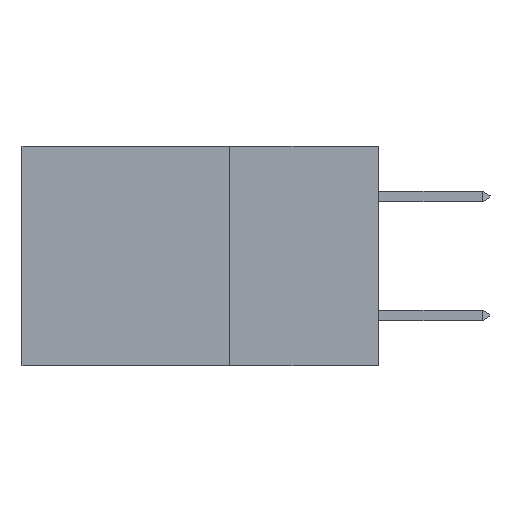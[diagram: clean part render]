
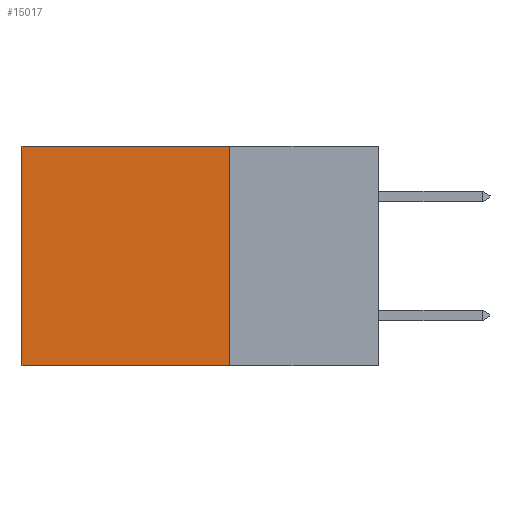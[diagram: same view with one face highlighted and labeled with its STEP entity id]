
A CAD part, left-side view. The second image highlights one B-rep face of the part: STEP entity #15017.
In plain terms, the highlighted planar face has unit normal (-1, 0, 0).
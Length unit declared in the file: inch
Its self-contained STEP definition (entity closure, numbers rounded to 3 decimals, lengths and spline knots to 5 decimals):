
#1255 = CARTESIAN_POINT ( 'NONE',  ( 0.2615, 0.6, -0.37 ) ) ;
#1549 = ORIENTED_EDGE ( 'NONE', *, *, #15933, .F. ) ;
#3287 = CARTESIAN_POINT ( 'NONE',  ( 0.2615, 0.6, 0. ) ) ;
#3736 = VERTEX_POINT ( 'NONE', #17501 ) ;
#4346 = VECTOR ( 'NONE', #14402, 39.37008 ) ;
#4404 = LINE ( 'NONE', #11683, #4346 ) ;
#4948 = EDGE_CURVE ( 'NONE', #3736, #9609, #12478, .T. ) ;
#5705 = EDGE_LOOP ( 'NONE', ( #17864, #1549, #15729, #14238 ) ) ;
#5894 = DIRECTION ( 'NONE',  ( 1., 0., 0. ) ) ;
#7299 = CARTESIAN_POINT ( 'NONE',  ( 0.2615, 0.25, -0.37 ) ) ;
#7676 = EDGE_CURVE ( 'NONE', #3736, #17178, #4404, .T. ) ;
#8292 = CARTESIAN_POINT ( 'NONE',  ( 0.2615, 0.25, 0. ) ) ;
#8500 = CARTESIAN_POINT ( 'NONE',  ( 0.2615, 0.25, -0.37 ) ) ;
#8706 = FACE_OUTER_BOUND ( 'NONE', #5705, .T. ) ;
#9117 = LINE ( 'NONE', #10249, #13138 ) ;
#9609 = VERTEX_POINT ( 'NONE', #3287 ) ;
#10249 = CARTESIAN_POINT ( 'NONE',  ( 0.2615, 0.25, -0.37 ) ) ;
#10652 = LINE ( 'NONE', #12328, #11546 ) ;
#10745 = DIRECTION ( 'NONE',  ( 0., 0., -1. ) ) ;
#11460 = EDGE_CURVE ( 'NONE', #9609, #15410, #10652, .T. ) ;
#11546 = VECTOR ( 'NONE', #10745, 39.37008 ) ;
#11683 = CARTESIAN_POINT ( 'NONE',  ( 0.2615, 0.25, -0.37 ) ) ;
#12328 = CARTESIAN_POINT ( 'NONE',  ( 0.2615, 0.6, -0.37 ) ) ;
#12478 = LINE ( 'NONE', #8292, #17111 ) ;
#12896 = DIRECTION ( 'NONE',  ( 0., 0., -1. ) ) ;
#13138 = VECTOR ( 'NONE', #14911, 39.37008 ) ;
#13408 = AXIS2_PLACEMENT_3D ( 'NONE', #7299, #5894, #12896 ) ;
#14238 = ORIENTED_EDGE ( 'NONE', *, *, #4948, .T. ) ;
#14402 = DIRECTION ( 'NONE',  ( 0., 0., -1. ) ) ;
#14911 = DIRECTION ( 'NONE',  ( 0., 1., 0. ) ) ;
#15017 = ADVANCED_FACE ( 'NONE', ( #8706 ), #17397, .F. ) ;
#15410 = VERTEX_POINT ( 'NONE', #1255 ) ;
#15729 = ORIENTED_EDGE ( 'NONE', *, *, #7676, .F. ) ;
#15933 = EDGE_CURVE ( 'NONE', #17178, #15410, #9117, .T. ) ;
#17111 = VECTOR ( 'NONE', #18303, 39.37008 ) ;
#17178 = VERTEX_POINT ( 'NONE', #8500 ) ;
#17397 = PLANE ( 'NONE',  #13408 ) ;
#17501 = CARTESIAN_POINT ( 'NONE',  ( 0.2615, 0.25, 0. ) ) ;
#17864 = ORIENTED_EDGE ( 'NONE', *, *, #11460, .T. ) ;
#18303 = DIRECTION ( 'NONE',  ( 0., 1., 0. ) ) ;
